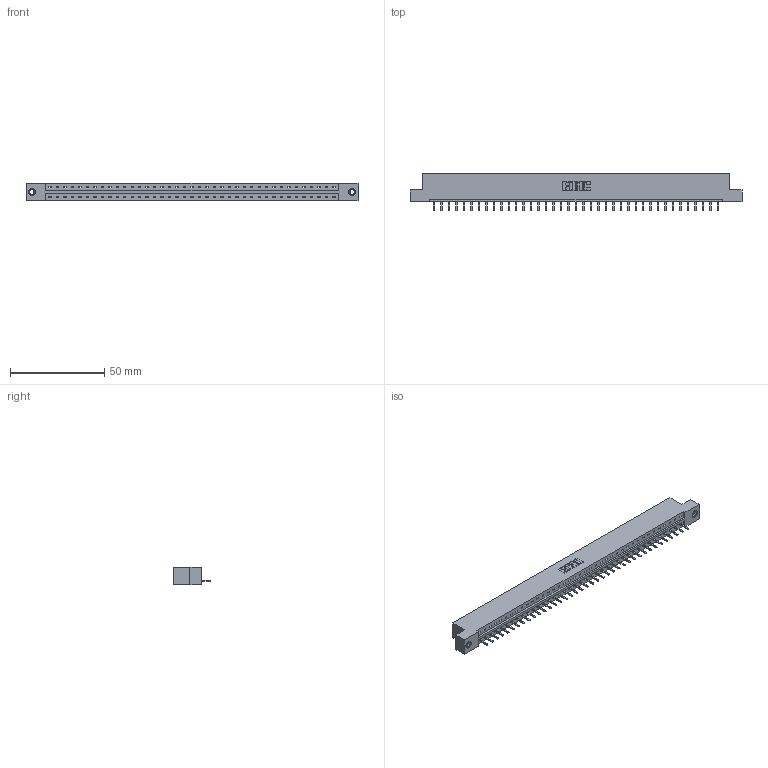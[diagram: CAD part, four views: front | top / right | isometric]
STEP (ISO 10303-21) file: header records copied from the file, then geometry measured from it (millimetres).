
FILE_DESCRIPTION (( 'STEP AP203' ), '1' );
FILE_NAME ('333-039-520-108.STEP', '2018-08-03T12:28:39', ( '' ), ( '' ), 'SwSTEP 2.0', 'SolidWorks 2016', '' );
FILE_SCHEMA (( 'CONFIG_CONTROL_DESIGN' ));
Length unit declared in the file: inch
Products named in the file (4): 333 Part_Flush - .156 Dia - TI; 345-292-001_345-293-120; 345-250-001_345-250-003-102; 333-039-520-108
Assembly tree (42 placements, depth 2):
  333-039-520-108
    333 Part_Flush - .156 Dia - TI
    345-292-001_345-293-120  x39
    345-250-001_345-250-003-102  x2
Bounding box: 176.07 x 20.02 x 9.4 mm (x, y, z)
Volume: 17573.4 mm3; surface area: 18626.8 mm2
Topology: 42 solids, 42 shells, 2592 faces, 7623 edges, 4970 vertices
Faces by surface type: plane 1818, cylinder 758, cone 12, torus 4
Entity records: 25530 total; most frequent: CARTESIAN_POINT 4398, ORIENTED_EDGE 4354, DIRECTION 3737, EDGE_CURVE 2177, LINE 2025, VECTOR 2025, VERTEX_POINT 1444, AXIS2_PLACEMENT_3D 856
